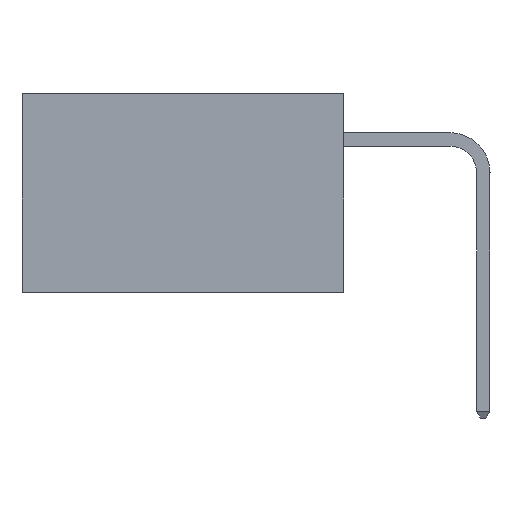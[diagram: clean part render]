
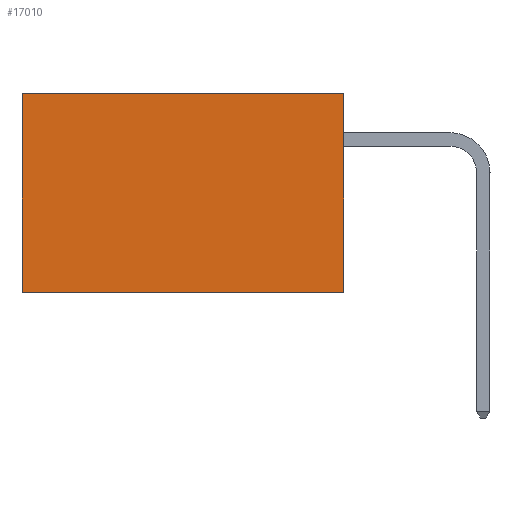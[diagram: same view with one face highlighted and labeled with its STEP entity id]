
A CAD part, left-side view. The second image highlights one B-rep face of the part: STEP entity #17010.
In plain terms, the highlighted planar face has unit normal (-1, 0, 0).
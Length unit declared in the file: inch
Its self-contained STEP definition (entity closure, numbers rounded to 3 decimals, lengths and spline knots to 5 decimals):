
#86 = LINE ( 'NONE', #6748, #18166 ) ;
#293 = CARTESIAN_POINT ( 'NONE',  ( 0.298, 0., 0. ) ) ;
#1695 = DIRECTION ( 'NONE',  ( 0., 0., -1. ) ) ;
#5021 = ORIENTED_EDGE ( 'NONE', *, *, #11703, .T. ) ;
#6748 = CARTESIAN_POINT ( 'NONE',  ( 0.298, 0., 0. ) ) ;
#6894 = AXIS2_PLACEMENT_3D ( 'NONE', #14979, #21028, #1695 ) ;
#6899 = DIRECTION ( 'NONE',  ( 0., 0., -1. ) ) ;
#7551 = CARTESIAN_POINT ( 'NONE',  ( 0.298, 0., -0.37 ) ) ;
#7606 = VERTEX_POINT ( 'NONE', #9745 ) ;
#9401 = CARTESIAN_POINT ( 'NONE',  ( 0.298, 0.6, -0.37 ) ) ;
#9711 = LINE ( 'NONE', #7551, #13636 ) ;
#9745 = CARTESIAN_POINT ( 'NONE',  ( 0.298, 0.6, 0. ) ) ;
#10126 = EDGE_LOOP ( 'NONE', ( #17132, #13681, #20426, #5021 ) ) ;
#10483 = VECTOR ( 'NONE', #27281, 39.37008 ) ;
#10902 = VECTOR ( 'NONE', #27321, 39.37008 ) ;
#10976 = EDGE_CURVE ( 'NONE', #7606, #11612, #21025, .T. ) ;
#11274 = EDGE_CURVE ( 'NONE', #28555, #11612, #9711, .T. ) ;
#11612 = VERTEX_POINT ( 'NONE', #9401 ) ;
#11703 = EDGE_CURVE ( 'NONE', #19817, #7606, #16021, .T. ) ;
#13636 = VECTOR ( 'NONE', #17706, 39.37008 ) ;
#13681 = ORIENTED_EDGE ( 'NONE', *, *, #11274, .F. ) ;
#14411 = CARTESIAN_POINT ( 'NONE',  ( 0.298, 0., 0. ) ) ;
#14979 = CARTESIAN_POINT ( 'NONE',  ( 0.298, 0., 0. ) ) ;
#16021 = LINE ( 'NONE', #293, #10902 ) ;
#17010 = ADVANCED_FACE ( 'NONE', ( #28153 ), #21323, .F. ) ;
#17132 = ORIENTED_EDGE ( 'NONE', *, *, #10976, .T. ) ;
#17706 = DIRECTION ( 'NONE',  ( 0., 1., 0. ) ) ;
#18166 = VECTOR ( 'NONE', #6899, 39.37008 ) ;
#19448 = CARTESIAN_POINT ( 'NONE',  ( 0.298, 0., -0.37 ) ) ;
#19817 = VERTEX_POINT ( 'NONE', #14411 ) ;
#20426 = ORIENTED_EDGE ( 'NONE', *, *, #24390, .F. ) ;
#21025 = LINE ( 'NONE', #22936, #10483 ) ;
#21028 = DIRECTION ( 'NONE',  ( 1., 0., 0. ) ) ;
#21323 = PLANE ( 'NONE',  #6894 ) ;
#22936 = CARTESIAN_POINT ( 'NONE',  ( 0.298, 0.6, 0. ) ) ;
#24390 = EDGE_CURVE ( 'NONE', #19817, #28555, #86, .T. ) ;
#27281 = DIRECTION ( 'NONE',  ( 0., 0., -1. ) ) ;
#27321 = DIRECTION ( 'NONE',  ( 0., 1., 0. ) ) ;
#28153 = FACE_OUTER_BOUND ( 'NONE', #10126, .T. ) ;
#28555 = VERTEX_POINT ( 'NONE', #19448 ) ;
